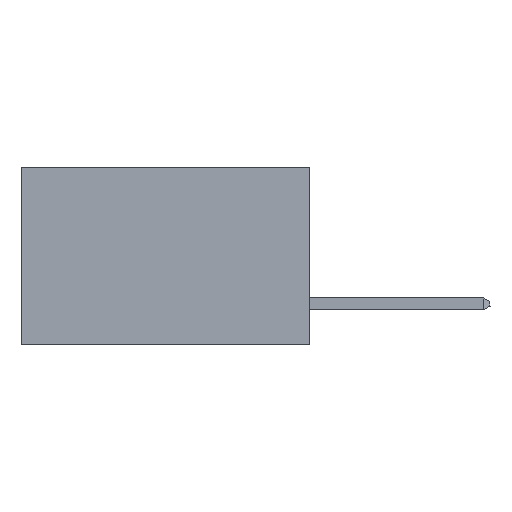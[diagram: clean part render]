
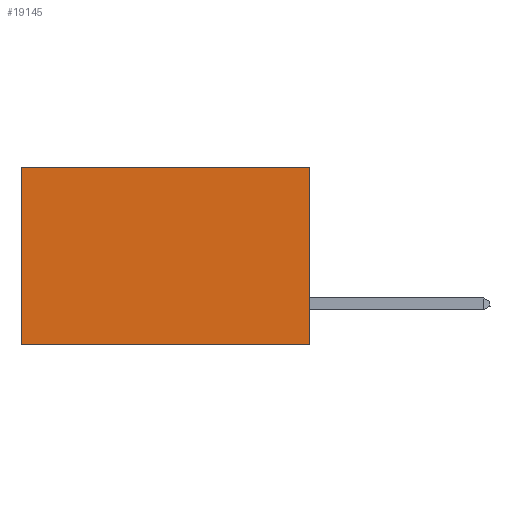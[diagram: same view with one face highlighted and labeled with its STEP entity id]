
A CAD part, left-side view. The second image highlights one B-rep face of the part: STEP entity #19145.
In plain terms, the highlighted planar face has unit normal (-1, 0, 0).
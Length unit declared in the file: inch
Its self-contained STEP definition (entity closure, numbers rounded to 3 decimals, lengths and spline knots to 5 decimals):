
#85 = AXIS2_PLACEMENT_3D ( 'NONE', #741, #10069, #17015 ) ;
#414 = VERTEX_POINT ( 'NONE', #23279 ) ;
#439 = CARTESIAN_POINT ( 'NONE',  ( 0.2875, 0.6, -0.37 ) ) ;
#593 = CARTESIAN_POINT ( 'NONE',  ( 0.2875, 0.6, 0. ) ) ;
#741 = CARTESIAN_POINT ( 'NONE',  ( 0.2875, 0., 0. ) ) ;
#1573 = ORIENTED_EDGE ( 'NONE', *, *, #19725, .T. ) ;
#1793 = VERTEX_POINT ( 'NONE', #439 ) ;
#2131 = VECTOR ( 'NONE', #15138, 39.37008 ) ;
#5586 = CARTESIAN_POINT ( 'NONE',  ( 0.2875, 0., 0. ) ) ;
#6489 = CARTESIAN_POINT ( 'NONE',  ( 0.2875, 0., -0.37 ) ) ;
#6513 = EDGE_CURVE ( 'NONE', #22100, #414, #7731, .T. ) ;
#6830 = CARTESIAN_POINT ( 'NONE',  ( 0.2875, 0., 0. ) ) ;
#7731 = LINE ( 'NONE', #6830, #17006 ) ;
#8288 = CARTESIAN_POINT ( 'NONE',  ( 0.2875, 0.6, 0. ) ) ;
#9533 = ORIENTED_EDGE ( 'NONE', *, *, #6513, .F. ) ;
#9858 = PLANE ( 'NONE',  #85 ) ;
#10069 = DIRECTION ( 'NONE',  ( 1., 0., 0. ) ) ;
#10262 = EDGE_CURVE ( 'NONE', #414, #1793, #10950, .T. ) ;
#10950 = LINE ( 'NONE', #6489, #14277 ) ;
#13220 = DIRECTION ( 'NONE',  ( 0., 1., 0. ) ) ;
#14277 = VECTOR ( 'NONE', #13220, 39.37008 ) ;
#14795 = FACE_OUTER_BOUND ( 'NONE', #17989, .T. ) ;
#14821 = EDGE_CURVE ( 'NONE', #22100, #26950, #15530, .T. ) ;
#15138 = DIRECTION ( 'NONE',  ( 0., 1., 0. ) ) ;
#15530 = LINE ( 'NONE', #5586, #2131 ) ;
#17006 = VECTOR ( 'NONE', #21416, 39.37008 ) ;
#17015 = DIRECTION ( 'NONE',  ( 0., 0., -1. ) ) ;
#17989 = EDGE_LOOP ( 'NONE', ( #1573, #18084, #9533, #29828 ) ) ;
#18084 = ORIENTED_EDGE ( 'NONE', *, *, #10262, .F. ) ;
#19145 = ADVANCED_FACE ( 'NONE', ( #14795 ), #9858, .F. ) ;
#19598 = VECTOR ( 'NONE', #24216, 39.37008 ) ;
#19725 = EDGE_CURVE ( 'NONE', #26950, #1793, #25918, .T. ) ;
#21416 = DIRECTION ( 'NONE',  ( 0., 0., -1. ) ) ;
#22100 = VERTEX_POINT ( 'NONE', #28715 ) ;
#23279 = CARTESIAN_POINT ( 'NONE',  ( 0.2875, 0., -0.37 ) ) ;
#24216 = DIRECTION ( 'NONE',  ( 0., 0., -1. ) ) ;
#25918 = LINE ( 'NONE', #593, #19598 ) ;
#26950 = VERTEX_POINT ( 'NONE', #8288 ) ;
#28715 = CARTESIAN_POINT ( 'NONE',  ( 0.2875, 0., 0. ) ) ;
#29828 = ORIENTED_EDGE ( 'NONE', *, *, #14821, .T. ) ;
